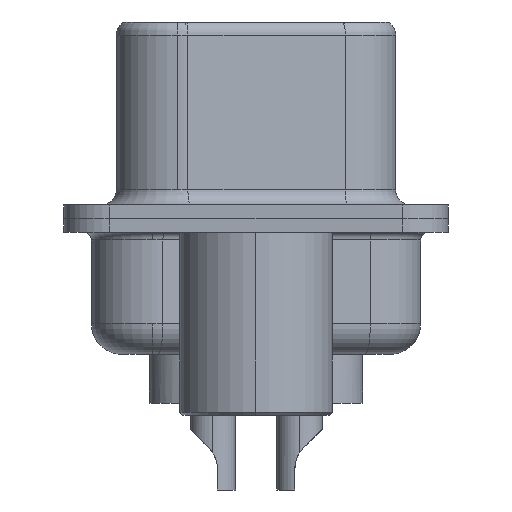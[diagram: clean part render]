
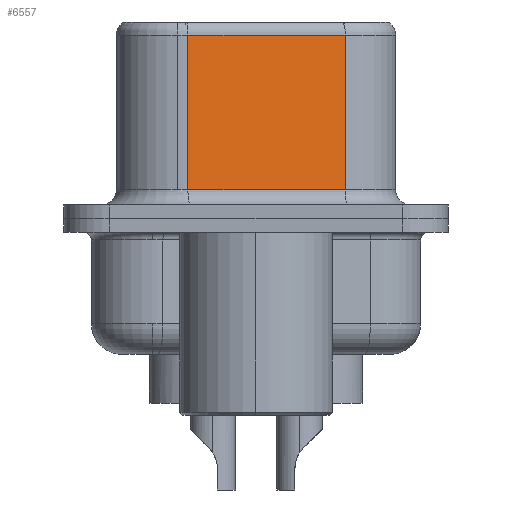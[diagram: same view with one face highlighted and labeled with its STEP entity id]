
A CAD part, left-side view. The second image highlights one B-rep face of the part: STEP entity #6557.
In plain terms, the highlighted planar face has unit normal (-0.985, -0.174, 0).
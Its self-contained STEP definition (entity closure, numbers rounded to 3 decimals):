
#2472 = VECTOR ( 'NONE', #26852, 1000. ) ;
#3045 = VECTOR ( 'NONE', #6078, 1000. ) ;
#3991 = LINE ( 'NONE', #14881, #3045 ) ;
#4437 = VERTEX_POINT ( 'NONE', #5329 ) ;
#4901 = VERTEX_POINT ( 'NONE', #8970 ) ;
#5262 = ORIENTED_EDGE ( 'NONE', *, *, #13770, .T. ) ;
#5329 = CARTESIAN_POINT ( 'NONE',  ( 4.58, -2.927, 6.02 ) ) ;
#6078 = DIRECTION ( 'NONE',  ( 0., 0., -1. ) ) ;
#6275 = CARTESIAN_POINT ( 'NONE',  ( 4.58, -2.927, 6.52 ) ) ;
#6375 = VECTOR ( 'NONE', #14834, 1000. ) ;
#6557 = ADVANCED_FACE ( 'NONE', ( #14943 ), #20828, .F. ) ;
#7227 = ORIENTED_EDGE ( 'NONE', *, *, #22979, .T. ) ;
#8246 = DIRECTION ( 'NONE',  ( -0.174, 0.985, 0. ) ) ;
#8970 = CARTESIAN_POINT ( 'NONE',  ( 3.67, 2.233, 6.02 ) ) ;
#9496 = EDGE_CURVE ( 'NONE', #4901, #11052, #27431, .T. ) ;
#9516 = CARTESIAN_POINT ( 'NONE',  ( 4.58, -2.927, 0.95 ) ) ;
#9852 = CARTESIAN_POINT ( 'NONE',  ( 4.58, -2.927, 6.02 ) ) ;
#10180 = ORIENTED_EDGE ( 'NONE', *, *, #9496, .T. ) ;
#11052 = VERTEX_POINT ( 'NONE', #17797 ) ;
#12091 = LINE ( 'NONE', #9852, #22306 ) ;
#13121 = EDGE_CURVE ( 'NONE', #4437, #25970, #3991, .T. ) ;
#13770 = EDGE_CURVE ( 'NONE', #4437, #4901, #12091, .T. ) ;
#14834 = DIRECTION ( 'NONE',  ( 0., 0., -1. ) ) ;
#14875 = EDGE_LOOP ( 'NONE', ( #19444, #5262, #10180, #7227 ) ) ;
#14881 = CARTESIAN_POINT ( 'NONE',  ( 4.58, -2.927, 6.52 ) ) ;
#14943 = FACE_OUTER_BOUND ( 'NONE', #14875, .T. ) ;
#17797 = CARTESIAN_POINT ( 'NONE',  ( 3.67, 2.233, 0.95 ) ) ;
#18094 = DIRECTION ( 'NONE',  ( -0.174, 0.985, 0. ) ) ;
#19444 = ORIENTED_EDGE ( 'NONE', *, *, #13121, .F. ) ;
#20828 = PLANE ( 'NONE',  #25482 ) ;
#22306 = VECTOR ( 'NONE', #18094, 1000. ) ;
#22979 = EDGE_CURVE ( 'NONE', #11052, #25970, #24345, .T. ) ;
#23646 = CARTESIAN_POINT ( 'NONE',  ( 3.67, 2.233, 6.52 ) ) ;
#24345 = LINE ( 'NONE', #9516, #2472 ) ;
#25308 = DIRECTION ( 'NONE',  ( 0.985, 0.174, 0. ) ) ;
#25482 = AXIS2_PLACEMENT_3D ( 'NONE', #6275, #25308, #8246 ) ;
#25970 = VERTEX_POINT ( 'NONE', #27364 ) ;
#26852 = DIRECTION ( 'NONE',  ( 0.174, -0.985, 0. ) ) ;
#27364 = CARTESIAN_POINT ( 'NONE',  ( 4.58, -2.927, 0.95 ) ) ;
#27431 = LINE ( 'NONE', #23646, #6375 ) ;
